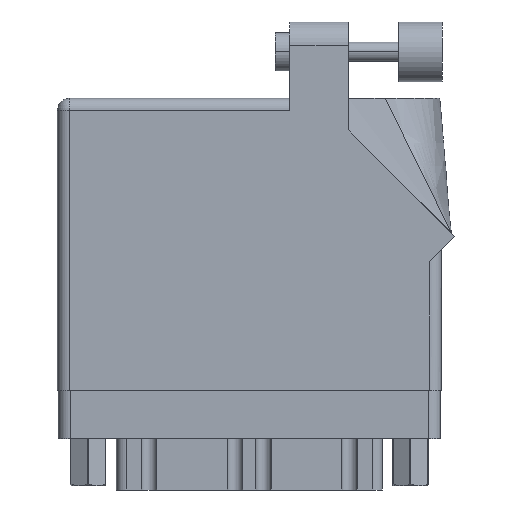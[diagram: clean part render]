
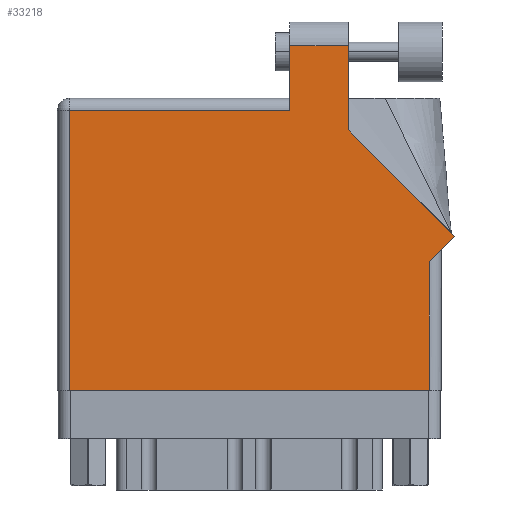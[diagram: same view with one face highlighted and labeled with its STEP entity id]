
A CAD part, front view. The second image highlights one B-rep face of the part: STEP entity #33218.
In plain terms, the highlighted face is planar.
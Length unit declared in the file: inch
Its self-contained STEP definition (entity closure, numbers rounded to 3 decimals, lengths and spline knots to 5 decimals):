
#286 = LINE ( 'NONE', #766, #18426 ) ;
#573 = VECTOR ( 'NONE', #17504, 39.37008 ) ;
#766 = CARTESIAN_POINT ( 'NONE',  ( 2.08071, 0.80771, 0. ) ) ;
#1315 = CARTESIAN_POINT ( 'NONE',  ( 0.062, 0., 0. ) ) ;
#2078 = CARTESIAN_POINT ( 'NONE',  ( 1.524, 1.36442, 0. ) ) ;
#2580 = ORIENTED_EDGE ( 'NONE', *, *, #14283, .T. ) ;
#3083 = LINE ( 'NONE', #20630, #573 ) ;
#3520 = LINE ( 'NONE', #18176, #11462 ) ;
#5424 = DIRECTION ( 'NONE',  ( 0., 1., 0. ) ) ;
#5885 = EDGE_CURVE ( 'NONE', #14775, #33159, #35763, .T. ) ;
#6980 = EDGE_CURVE ( 'NONE', #30793, #11854, #286, .T. ) ;
#7793 = CARTESIAN_POINT ( 'NONE',  ( 1.948, 0., 0. ) ) ;
#8193 = VECTOR ( 'NONE', #26082, 39.37008 ) ;
#8271 = PLANE ( 'NONE',  #21101 ) ;
#9241 = VERTEX_POINT ( 'NONE', #19683 ) ;
#10265 = VECTOR ( 'NONE', #5424, 39.37008 ) ;
#11462 = VECTOR ( 'NONE', #15274, 39.37008 ) ;
#11854 = VERTEX_POINT ( 'NONE', #14657 ) ;
#11875 = DIRECTION ( 'NONE',  ( 0., 0., -1. ) ) ;
#11932 = CARTESIAN_POINT ( 'NONE',  ( 1.217, 1.805, 0. ) ) ;
#13479 = CARTESIAN_POINT ( 'NONE',  ( 0.062, 1.468, 0. ) ) ;
#14152 = LINE ( 'NONE', #40301, #22288 ) ;
#14283 = EDGE_CURVE ( 'NONE', #33159, #36397, #43052, .T. ) ;
#14657 = CARTESIAN_POINT ( 'NONE',  ( 1.524, 1.36442, 0. ) ) ;
#14704 = CARTESIAN_POINT ( 'NONE',  ( 0., 0., 0. ) ) ;
#14775 = VERTEX_POINT ( 'NONE', #13479 ) ;
#14903 = DIRECTION ( 'NONE',  ( -0.707, 0.707, 0. ) ) ;
#15274 = DIRECTION ( 'NONE',  ( -1., 0., 0. ) ) ;
#16371 = ORIENTED_EDGE ( 'NONE', *, *, #40241, .T. ) ;
#17356 = ORIENTED_EDGE ( 'NONE', *, *, #26858, .T. ) ;
#17504 = DIRECTION ( 'NONE',  ( 0.707, 0.707, 0. ) ) ;
#18176 = CARTESIAN_POINT ( 'NONE',  ( 1.217, 1.805, 0. ) ) ;
#18426 = VECTOR ( 'NONE', #14903, 39.37008 ) ;
#19099 = CARTESIAN_POINT ( 'NONE',  ( 0., 1.468, 0. ) ) ;
#19683 = CARTESIAN_POINT ( 'NONE',  ( 1.948, 0.675, 0. ) ) ;
#20138 = CARTESIAN_POINT ( 'NONE',  ( 1.524, 1.805, 0. ) ) ;
#20629 = EDGE_CURVE ( 'NONE', #37203, #14775, #22698, .T. ) ;
#20630 = CARTESIAN_POINT ( 'NONE',  ( 2.01, 0.737, 0. ) ) ;
#21101 = AXIS2_PLACEMENT_3D ( 'NONE', #44995, #11875, #37072 ) ;
#21170 = CARTESIAN_POINT ( 'NONE',  ( 2.08071, 0.80771, 0. ) ) ;
#22288 = VECTOR ( 'NONE', #29039, 39.37008 ) ;
#22698 = LINE ( 'NONE', #19099, #8193 ) ;
#24061 = LINE ( 'NONE', #24782, #25313 ) ;
#24142 = ORIENTED_EDGE ( 'NONE', *, *, #5885, .T. ) ;
#24594 = EDGE_LOOP ( 'NONE', ( #26326, #16371, #17356, #34106, #24142, #2580, #28639, #35996, #25611 ) ) ;
#24782 = CARTESIAN_POINT ( 'NONE',  ( 1.948, 0.737, 0. ) ) ;
#25313 = VECTOR ( 'NONE', #27909, 39.37008 ) ;
#25563 = EDGE_CURVE ( 'NONE', #36397, #9241, #24061, .T. ) ;
#25611 = ORIENTED_EDGE ( 'NONE', *, *, #6980, .T. ) ;
#26082 = DIRECTION ( 'NONE',  ( -1., 0., 0. ) ) ;
#26326 = ORIENTED_EDGE ( 'NONE', *, *, #44567, .T. ) ;
#26858 = EDGE_CURVE ( 'NONE', #32908, #37203, #14152, .T. ) ;
#27909 = DIRECTION ( 'NONE',  ( 0., 1., 0. ) ) ;
#28639 = ORIENTED_EDGE ( 'NONE', *, *, #25563, .T. ) ;
#29039 = DIRECTION ( 'NONE',  ( 0., -1., 0. ) ) ;
#30660 = LINE ( 'NONE', #2078, #10265 ) ;
#30793 = VERTEX_POINT ( 'NONE', #21170 ) ;
#32481 = DIRECTION ( 'NONE',  ( 1., 0., 0. ) ) ;
#32664 = CARTESIAN_POINT ( 'NONE',  ( 1.217, 1.468, 0. ) ) ;
#32908 = VERTEX_POINT ( 'NONE', #11932 ) ;
#33159 = VERTEX_POINT ( 'NONE', #1315 ) ;
#33218 = ADVANCED_FACE ( 'NONE', ( #40684 ), #8271, .F. ) ;
#34106 = ORIENTED_EDGE ( 'NONE', *, *, #20629, .T. ) ;
#35656 = EDGE_CURVE ( 'NONE', #9241, #30793, #3083, .T. ) ;
#35763 = LINE ( 'NONE', #43184, #46714 ) ;
#35996 = ORIENTED_EDGE ( 'NONE', *, *, #35656, .T. ) ;
#36397 = VERTEX_POINT ( 'NONE', #7793 ) ;
#37072 = DIRECTION ( 'NONE',  ( -1., 0., 0. ) ) ;
#37203 = VERTEX_POINT ( 'NONE', #32664 ) ;
#40241 = EDGE_CURVE ( 'NONE', #44228, #32908, #3520, .T. ) ;
#40301 = CARTESIAN_POINT ( 'NONE',  ( 1.217, 1.53, 0. ) ) ;
#40684 = FACE_OUTER_BOUND ( 'NONE', #24594, .T. ) ;
#42475 = VECTOR ( 'NONE', #32481, 39.37008 ) ;
#42725 = DIRECTION ( 'NONE',  ( 0., -1., 0. ) ) ;
#43052 = LINE ( 'NONE', #14704, #42475 ) ;
#43184 = CARTESIAN_POINT ( 'NONE',  ( 0.062, 0., 0. ) ) ;
#44228 = VERTEX_POINT ( 'NONE', #20138 ) ;
#44567 = EDGE_CURVE ( 'NONE', #11854, #44228, #30660, .T. ) ;
#44995 = CARTESIAN_POINT ( 'NONE',  ( 0., 1.53, 0. ) ) ;
#46714 = VECTOR ( 'NONE', #42725, 39.37008 ) ;
